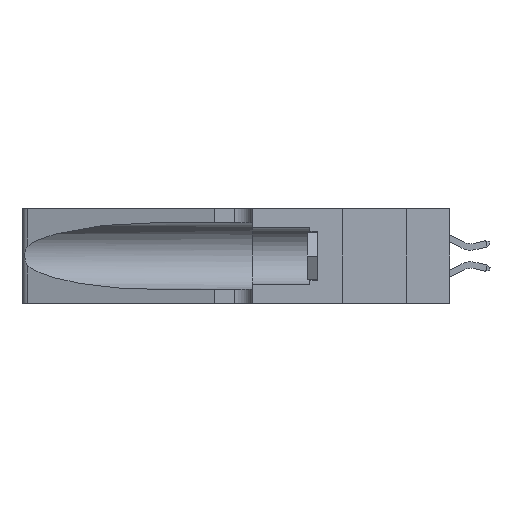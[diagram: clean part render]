
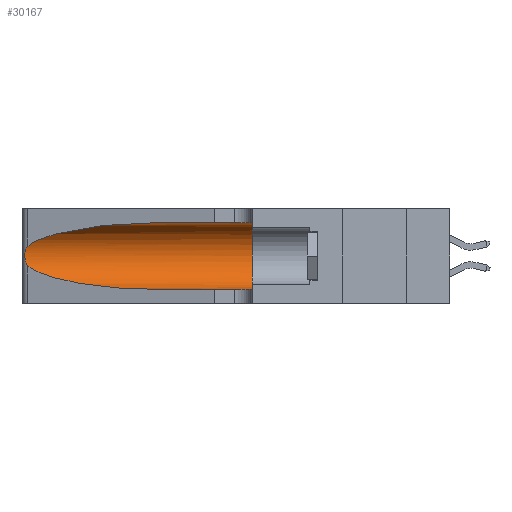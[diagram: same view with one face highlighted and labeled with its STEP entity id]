
A CAD part, left-side view. The second image highlights one B-rep face of the part: STEP entity #30167.
In plain terms, the highlighted cylindrical face has radius 3.308 mm (diameter 6.617 mm), a partial arc.
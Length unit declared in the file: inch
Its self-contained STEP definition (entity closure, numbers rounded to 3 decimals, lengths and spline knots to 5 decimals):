
#43 = CARTESIAN_POINT ( 'NONE',  ( 0.1305, 0.72297, 0.31525 ) ) ;
#1362 = CARTESIAN_POINT ( 'NONE',  ( 0.1305, 0.72297, 0.05475 ) ) ;
#1404 = ORIENTED_EDGE ( 'NONE', *, *, #21597, .T. ) ;
#2261 = VERTEX_POINT ( 'NONE', #6298 ) ;
#3591 = AXIS2_PLACEMENT_3D ( 'NONE', #22848, #6728, #30889 ) ;
#4233 = ORIENTED_EDGE ( 'NONE', *, *, #19525, .T. ) ;
#4697 = EDGE_CURVE ( 'NONE', #7588, #10151, #15645, .T. ) ;
#4732 = CARTESIAN_POINT ( 'NONE',  ( 0.1305, 0.35, 0.31525 ) ) ;
#5145 = CARTESIAN_POINT ( 'NONE',  ( 0.18966, 0.96281, 0.05475 ) ) ;
#5586 = CARTESIAN_POINT ( 'NONE',  ( 0.25789, 1.23486, 0.15765 ) ) ;
#6298 = CARTESIAN_POINT ( 'NONE',  ( 0.1305, 0.35, 0.05475 ) ) ;
#6304 = AXIS2_PLACEMENT_3D ( 'NONE', #25359, #12014, #22629 ) ;
#6728 = DIRECTION ( 'NONE',  ( 0., -1., 0. ) ) ;
#6932 = CARTESIAN_POINT ( 'NONE',  ( 0.25854, 1.2359, 0.20912 ) ) ;
#7062 = CARTESIAN_POINT ( 'NONE',  ( 0.26017, 1.23833, 0.17102 ) ) ;
#7588 = VERTEX_POINT ( 'NONE', #31299 ) ;
#8300 = DIRECTION ( 'NONE',  ( 0., -1., 0. ) ) ;
#8909 = EDGE_CURVE ( 'NONE', #34780, #33419, #11914, .T. ) ;
#10151 = VERTEX_POINT ( 'NONE', #4732 ) ;
#10210 =( BOUNDED_CURVE ( )  B_SPLINE_CURVE ( 3, ( #13235, #26684, #5145, #21246 ),
 .UNSPECIFIED., .F., .F. ) 
 B_SPLINE_CURVE_WITH_KNOTS ( ( 4, 4 ),
 ( 3.44316, 4.71239 ),
 .UNSPECIFIED. ) 
 CURVE ( )  GEOMETRIC_REPRESENTATION_ITEM ( )  RATIONAL_B_SPLINE_CURVE ( ( 1., 0.87, 0.87, 1. ) ) 
 REPRESENTATION_ITEM ( '' )  );
#11914 = B_SPLINE_CURVE_WITH_KNOTS ( 'NONE', 3,
 ( #30045, #25454, #12576, #12694, #6932, #28393, #33832, #20486, #7062, #18240, #5586, #13442, #12975, #34594 ),
 .UNSPECIFIED., .F., .F.,
 ( 4, 2, 2, 2, 2, 2, 4 ),
 ( 0., 0.00027, 0.00053, 0.00107, 0.0016, 0.00187, 0.00214 ),
 .UNSPECIFIED. ) ;
#12014 = DIRECTION ( 'NONE',  ( 0., 1., 0. ) ) ;
#12576 = CARTESIAN_POINT ( 'NONE',  ( 0.25639, 1.23184, 0.21858 ) ) ;
#12694 = CARTESIAN_POINT ( 'NONE',  ( 0.25787, 1.23484, 0.2124 ) ) ;
#12975 = CARTESIAN_POINT ( 'NONE',  ( 0.25555, 1.22993, 0.14849 ) ) ;
#13235 = CARTESIAN_POINT ( 'NONE',  ( 0.25487, 1.22718, 0.14631 ) ) ;
#13442 = CARTESIAN_POINT ( 'NONE',  ( 0.25639, 1.23186, 0.15144 ) ) ;
#13851 = ORIENTED_EDGE ( 'NONE', *, *, #29903, .T. ) ;
#14092 = CARTESIAN_POINT ( 'NONE',  ( 0.25487, 1.22718, 0.22369 ) ) ;
#14378 = VECTOR ( 'NONE', #8300, 39.37008 ) ;
#15645 = LINE ( 'NONE', #32135, #14378 ) ;
#15857 = DIRECTION ( 'NONE',  ( 0., -1., 0. ) ) ;
#16466 = LINE ( 'NONE', #29046, #20224 ) ;
#18240 = CARTESIAN_POINT ( 'NONE',  ( 0.25856, 1.23593, 0.16098 ) ) ;
#19525 = EDGE_CURVE ( 'NONE', #22662, #2261, #16466, .T. ) ;
#19714 =( BOUNDED_CURVE ( )  B_SPLINE_CURVE ( 3, ( #43, #26916, #21714, #29728 ),
 .UNSPECIFIED., .F., .F. ) 
 B_SPLINE_CURVE_WITH_KNOTS ( ( 4, 4 ),
 ( 1.5708, 2.84003 ),
 .UNSPECIFIED. ) 
 CURVE ( )  GEOMETRIC_REPRESENTATION_ITEM ( )  RATIONAL_B_SPLINE_CURVE ( ( 1., 0.87, 0.87, 1. ) ) 
 REPRESENTATION_ITEM ( '' )  );
#20224 = VECTOR ( 'NONE', #15857, 39.37008 ) ;
#20486 = CARTESIAN_POINT ( 'NONE',  ( 0.26075, 1.23896, 0.178 ) ) ;
#20725 = CIRCLE ( 'NONE', #6304, 0.13025 ) ;
#21246 = CARTESIAN_POINT ( 'NONE',  ( 0.1305, 0.72297, 0.05475 ) ) ;
#21597 = EDGE_CURVE ( 'NONE', #33419, #22662, #10210, .T. ) ;
#21714 = CARTESIAN_POINT ( 'NONE',  ( 0.2373, 1.15595, 0.28018 ) ) ;
#22629 = DIRECTION ( 'NONE',  ( 0., 0., 1. ) ) ;
#22662 = VERTEX_POINT ( 'NONE', #1362 ) ;
#22848 = CARTESIAN_POINT ( 'NONE',  ( 0.1305, 1.61858, 0.185 ) ) ;
#24138 = FACE_OUTER_BOUND ( 'NONE', #25696, .T. ) ;
#24489 = EDGE_CURVE ( 'NONE', #10151, #2261, #20725, .T. ) ;
#25359 = CARTESIAN_POINT ( 'NONE',  ( 0.1305, 0.35, 0.185 ) ) ;
#25454 = CARTESIAN_POINT ( 'NONE',  ( 0.25555, 1.22994, 0.2215 ) ) ;
#25696 = EDGE_LOOP ( 'NONE', ( #13851, #30210, #1404, #4233, #31455, #28821 ) ) ;
#26684 = CARTESIAN_POINT ( 'NONE',  ( 0.2373, 1.15595, 0.08982 ) ) ;
#26916 = CARTESIAN_POINT ( 'NONE',  ( 0.18966, 0.96281, 0.31525 ) ) ;
#28393 = CARTESIAN_POINT ( 'NONE',  ( 0.26018, 1.23835, 0.19895 ) ) ;
#28821 = ORIENTED_EDGE ( 'NONE', *, *, #4697, .F. ) ;
#29046 = CARTESIAN_POINT ( 'NONE',  ( 0.1305, 1.61858, 0.05475 ) ) ;
#29728 = CARTESIAN_POINT ( 'NONE',  ( 0.25487, 1.22718, 0.22369 ) ) ;
#29814 = CARTESIAN_POINT ( 'NONE',  ( 0.25487, 1.22718, 0.14631 ) ) ;
#29903 = EDGE_CURVE ( 'NONE', #7588, #34780, #19714, .T. ) ;
#29945 = CYLINDRICAL_SURFACE ( 'NONE', #3591, 0.13025 ) ;
#30045 = CARTESIAN_POINT ( 'NONE',  ( 0.25487, 1.22718, 0.22369 ) ) ;
#30167 = ADVANCED_FACE ( 'NONE', ( #24138 ), #29945, .F. ) ;
#30210 = ORIENTED_EDGE ( 'NONE', *, *, #8909, .T. ) ;
#30889 = DIRECTION ( 'NONE',  ( 0., 0., -1. ) ) ;
#31299 = CARTESIAN_POINT ( 'NONE',  ( 0.1305, 0.72297, 0.31525 ) ) ;
#31455 = ORIENTED_EDGE ( 'NONE', *, *, #24489, .F. ) ;
#32135 = CARTESIAN_POINT ( 'NONE',  ( 0.1305, 1.61858, 0.31525 ) ) ;
#33419 = VERTEX_POINT ( 'NONE', #29814 ) ;
#33832 = CARTESIAN_POINT ( 'NONE',  ( 0.26075, 1.23896, 0.19203 ) ) ;
#34594 = CARTESIAN_POINT ( 'NONE',  ( 0.25487, 1.22718, 0.14631 ) ) ;
#34780 = VERTEX_POINT ( 'NONE', #14092 ) ;
